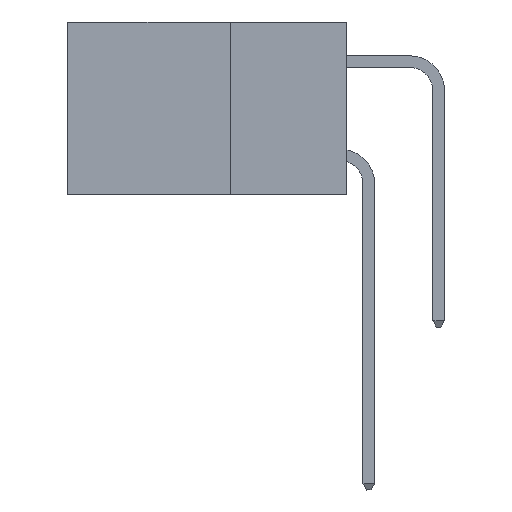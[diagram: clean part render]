
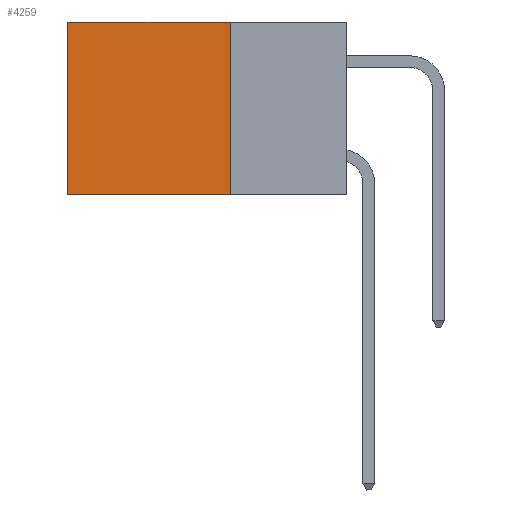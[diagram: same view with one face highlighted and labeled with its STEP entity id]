
A CAD part, left-side view. The second image highlights one B-rep face of the part: STEP entity #4259.
In plain terms, the highlighted planar face has unit normal (-1, 0, 0).
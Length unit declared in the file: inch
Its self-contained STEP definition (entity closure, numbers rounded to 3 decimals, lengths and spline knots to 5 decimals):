
#452 = CARTESIAN_POINT ( 'NONE',  ( 0.2875, 0.25, 0. ) ) ;
#611 = EDGE_CURVE ( 'NONE', #2124, #25945, #5162, .T. ) ;
#2124 = VERTEX_POINT ( 'NONE', #24190 ) ;
#2559 = VERTEX_POINT ( 'NONE', #14648 ) ;
#3620 = LINE ( 'NONE', #22255, #27942 ) ;
#4243 = LINE ( 'NONE', #7551, #5282 ) ;
#4259 = ADVANCED_FACE ( 'NONE', ( #17064 ), #22292, .F. ) ;
#4752 = DIRECTION ( 'NONE',  ( 0., 1., 0. ) ) ;
#5162 = LINE ( 'NONE', #452, #20401 ) ;
#5282 = VECTOR ( 'NONE', #20542, 39.37008 ) ;
#5336 = EDGE_CURVE ( 'NONE', #2559, #26655, #21457, .T. ) ;
#5933 = ORIENTED_EDGE ( 'NONE', *, *, #5336, .T. ) ;
#6681 = ORIENTED_EDGE ( 'NONE', *, *, #24189, .T. ) ;
#7551 = CARTESIAN_POINT ( 'NONE',  ( 0.2875, 0.25, -0.37 ) ) ;
#8987 = CARTESIAN_POINT ( 'NONE',  ( 0.2875, 0.25, 0. ) ) ;
#10038 = CARTESIAN_POINT ( 'NONE',  ( 0.2875, 0.25, -0.37 ) ) ;
#11209 = DIRECTION ( 'NONE',  ( 0., 0., -1. ) ) ;
#12735 = EDGE_CURVE ( 'NONE', #25945, #26655, #4243, .T. ) ;
#13411 = AXIS2_PLACEMENT_3D ( 'NONE', #8987, #15884, #11209 ) ;
#14648 = CARTESIAN_POINT ( 'NONE',  ( 0.2875, 0.6, 0. ) ) ;
#14738 = ORIENTED_EDGE ( 'NONE', *, *, #611, .F. ) ;
#14869 = VECTOR ( 'NONE', #19207, 39.37008 ) ;
#15884 = DIRECTION ( 'NONE',  ( 1., 0., 0. ) ) ;
#16350 = EDGE_LOOP ( 'NONE', ( #5933, #19021, #14738, #6681 ) ) ;
#17064 = FACE_OUTER_BOUND ( 'NONE', #16350, .T. ) ;
#19021 = ORIENTED_EDGE ( 'NONE', *, *, #12735, .F. ) ;
#19207 = DIRECTION ( 'NONE',  ( 0., 0., -1. ) ) ;
#20401 = VECTOR ( 'NONE', #26231, 39.37008 ) ;
#20542 = DIRECTION ( 'NONE',  ( 0., 1., 0. ) ) ;
#21457 = LINE ( 'NONE', #23662, #14869 ) ;
#22255 = CARTESIAN_POINT ( 'NONE',  ( 0.2875, 0.25, 0. ) ) ;
#22292 = PLANE ( 'NONE',  #13411 ) ;
#23591 = CARTESIAN_POINT ( 'NONE',  ( 0.2875, 0.6, -0.37 ) ) ;
#23662 = CARTESIAN_POINT ( 'NONE',  ( 0.2875, 0.6, 0. ) ) ;
#24189 = EDGE_CURVE ( 'NONE', #2124, #2559, #3620, .T. ) ;
#24190 = CARTESIAN_POINT ( 'NONE',  ( 0.2875, 0.25, 0. ) ) ;
#25945 = VERTEX_POINT ( 'NONE', #10038 ) ;
#26231 = DIRECTION ( 'NONE',  ( 0., 0., -1. ) ) ;
#26655 = VERTEX_POINT ( 'NONE', #23591 ) ;
#27942 = VECTOR ( 'NONE', #4752, 39.37008 ) ;
